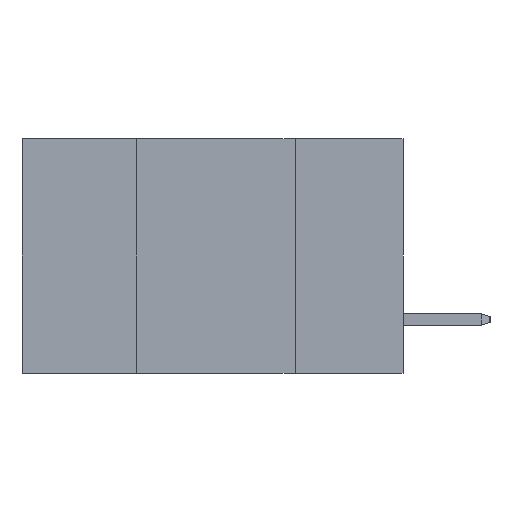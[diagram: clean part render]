
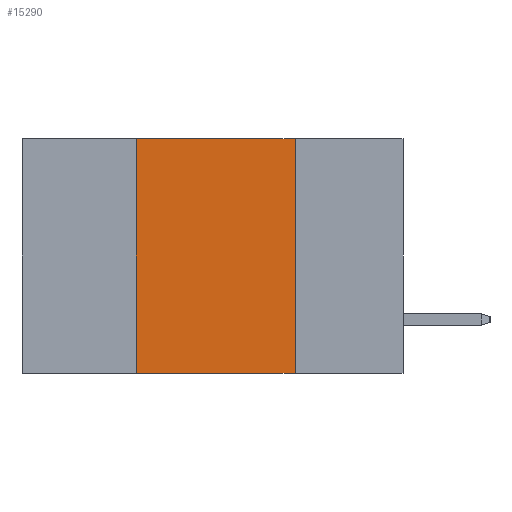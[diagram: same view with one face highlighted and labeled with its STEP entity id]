
A CAD part, left-side view. The second image highlights one B-rep face of the part: STEP entity #15290.
In plain terms, the highlighted planar face has unit normal (-1, 0, 0).
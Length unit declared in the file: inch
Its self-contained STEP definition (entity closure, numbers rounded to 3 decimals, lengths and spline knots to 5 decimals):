
#400 = CARTESIAN_POINT ( 'NONE',  ( 0., 0.42, 0. ) ) ;
#482 = DIRECTION ( 'NONE',  ( 0., -1., 0. ) ) ;
#856 = VECTOR ( 'NONE', #14395, 39.37008 ) ;
#1129 = LINE ( 'NONE', #14553, #856 ) ;
#1509 = ORIENTED_EDGE ( 'NONE', *, *, #7488, .F. ) ;
#1622 = LINE ( 'NONE', #14902, #4691 ) ;
#2867 = LINE ( 'NONE', #4147, #5706 ) ;
#3126 = VERTEX_POINT ( 'NONE', #15626 ) ;
#4147 = CARTESIAN_POINT ( 'NONE',  ( 0., 0.6, -0.37 ) ) ;
#4216 = AXIS2_PLACEMENT_3D ( 'NONE', #12438, #6045, #4846 ) ;
#4311 = CARTESIAN_POINT ( 'NONE',  ( 0., 0.17, 0. ) ) ;
#4691 = VECTOR ( 'NONE', #12145, 39.37008 ) ;
#4846 = DIRECTION ( 'NONE',  ( 0., 0., -1. ) ) ;
#5533 = VERTEX_POINT ( 'NONE', #400 ) ;
#5706 = VECTOR ( 'NONE', #482, 39.37008 ) ;
#6045 = DIRECTION ( 'NONE',  ( 1., 0., 0. ) ) ;
#6221 = ORIENTED_EDGE ( 'NONE', *, *, #8359, .T. ) ;
#7232 = VERTEX_POINT ( 'NONE', #10194 ) ;
#7378 = EDGE_LOOP ( 'NONE', ( #12748, #14084, #1509, #6221 ) ) ;
#7420 = FACE_OUTER_BOUND ( 'NONE', #7378, .T. ) ;
#7488 = EDGE_CURVE ( 'NONE', #7232, #5533, #1622, .T. ) ;
#7689 = CARTESIAN_POINT ( 'NONE',  ( 0., 0.6, 0. ) ) ;
#8359 = EDGE_CURVE ( 'NONE', #7232, #3126, #2867, .T. ) ;
#9751 = VERTEX_POINT ( 'NONE', #4311 ) ;
#10194 = CARTESIAN_POINT ( 'NONE',  ( 0., 0.42, -0.37 ) ) ;
#11299 = EDGE_CURVE ( 'NONE', #9751, #3126, #1129, .T. ) ;
#12145 = DIRECTION ( 'NONE',  ( 0., 0., 1. ) ) ;
#12438 = CARTESIAN_POINT ( 'NONE',  ( 0., 0.6, 0. ) ) ;
#12520 = PLANE ( 'NONE',  #4216 ) ;
#12701 = LINE ( 'NONE', #7689, #12717 ) ;
#12717 = VECTOR ( 'NONE', #12793, 39.37008 ) ;
#12748 = ORIENTED_EDGE ( 'NONE', *, *, #11299, .F. ) ;
#12793 = DIRECTION ( 'NONE',  ( 0., -1., 0. ) ) ;
#14084 = ORIENTED_EDGE ( 'NONE', *, *, #16746, .F. ) ;
#14395 = DIRECTION ( 'NONE',  ( 0., 0., -1. ) ) ;
#14553 = CARTESIAN_POINT ( 'NONE',  ( 0., 0.17, 0. ) ) ;
#14902 = CARTESIAN_POINT ( 'NONE',  ( 0., 0.42, 0. ) ) ;
#15290 = ADVANCED_FACE ( 'NONE', ( #7420 ), #12520, .F. ) ;
#15626 = CARTESIAN_POINT ( 'NONE',  ( 0., 0.17, -0.37 ) ) ;
#16746 = EDGE_CURVE ( 'NONE', #5533, #9751, #12701, .T. ) ;
